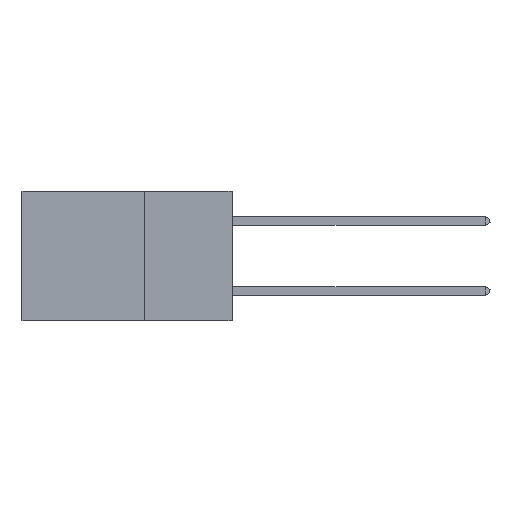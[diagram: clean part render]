
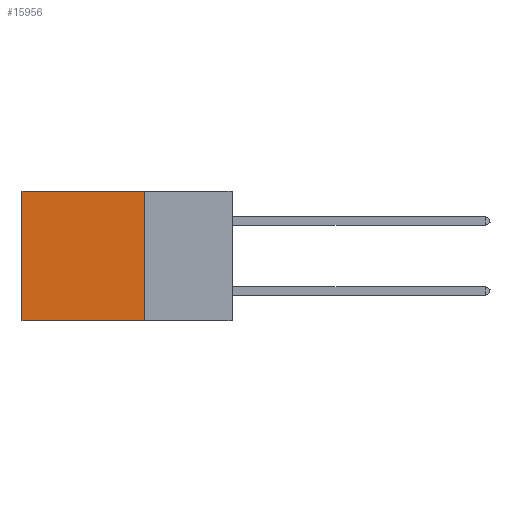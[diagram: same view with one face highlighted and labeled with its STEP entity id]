
A CAD part, left-side view. The second image highlights one B-rep face of the part: STEP entity #15956.
In plain terms, the highlighted planar face has unit normal (-1, 0, 0).
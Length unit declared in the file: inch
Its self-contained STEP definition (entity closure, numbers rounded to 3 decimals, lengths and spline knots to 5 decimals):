
#139 = DIRECTION ( 'NONE',  ( 1., 0., 0. ) ) ;
#235 = CARTESIAN_POINT ( 'NONE',  ( 0.2875, 0.6, -0.37 ) ) ;
#438 = ORIENTED_EDGE ( 'NONE', *, *, #8386, .T. ) ;
#819 = EDGE_CURVE ( 'NONE', #12470, #19053, #14861, .T. ) ;
#3284 = AXIS2_PLACEMENT_3D ( 'NONE', #11725, #139, #13626 ) ;
#4146 = VERTEX_POINT ( 'NONE', #8491 ) ;
#4432 = DIRECTION ( 'NONE',  ( 0., 1., 0. ) ) ;
#5366 = CARTESIAN_POINT ( 'NONE',  ( 0.2875, 0.25, 0. ) ) ;
#5460 = VERTEX_POINT ( 'NONE', #22839 ) ;
#5474 = EDGE_CURVE ( 'NONE', #5460, #4146, #20321, .T. ) ;
#5989 = CARTESIAN_POINT ( 'NONE',  ( 0.2875, 0.25, -0.37 ) ) ;
#6579 = VECTOR ( 'NONE', #16697, 39.37008 ) ;
#8058 = EDGE_CURVE ( 'NONE', #5460, #12470, #16604, .T. ) ;
#8386 = EDGE_CURVE ( 'NONE', #4146, #19053, #14556, .T. ) ;
#8491 = CARTESIAN_POINT ( 'NONE',  ( 0.2875, 0.6, 0. ) ) ;
#9884 = VECTOR ( 'NONE', #20819, 39.37008 ) ;
#10475 = DIRECTION ( 'NONE',  ( 0., 0., -1. ) ) ;
#11123 = FACE_OUTER_BOUND ( 'NONE', #21142, .T. ) ;
#11725 = CARTESIAN_POINT ( 'NONE',  ( 0.2875, 0.25, 0. ) ) ;
#12298 = ORIENTED_EDGE ( 'NONE', *, *, #5474, .T. ) ;
#12470 = VERTEX_POINT ( 'NONE', #18714 ) ;
#13626 = DIRECTION ( 'NONE',  ( 0., 0., -1. ) ) ;
#13695 = ORIENTED_EDGE ( 'NONE', *, *, #819, .F. ) ;
#14556 = LINE ( 'NONE', #17536, #22975 ) ;
#14861 = LINE ( 'NONE', #5989, #9884 ) ;
#15545 = ORIENTED_EDGE ( 'NONE', *, *, #8058, .F. ) ;
#15956 = ADVANCED_FACE ( 'NONE', ( #11123 ), #22588, .F. ) ;
#16145 = VECTOR ( 'NONE', #4432, 39.37008 ) ;
#16604 = LINE ( 'NONE', #5366, #6579 ) ;
#16697 = DIRECTION ( 'NONE',  ( 0., 0., -1. ) ) ;
#17536 = CARTESIAN_POINT ( 'NONE',  ( 0.2875, 0.6, 0. ) ) ;
#17645 = CARTESIAN_POINT ( 'NONE',  ( 0.2875, 0.25, 0. ) ) ;
#18714 = CARTESIAN_POINT ( 'NONE',  ( 0.2875, 0.25, -0.37 ) ) ;
#19053 = VERTEX_POINT ( 'NONE', #235 ) ;
#20321 = LINE ( 'NONE', #17645, #16145 ) ;
#20819 = DIRECTION ( 'NONE',  ( 0., 1., 0. ) ) ;
#21142 = EDGE_LOOP ( 'NONE', ( #438, #13695, #15545, #12298 ) ) ;
#22588 = PLANE ( 'NONE',  #3284 ) ;
#22839 = CARTESIAN_POINT ( 'NONE',  ( 0.2875, 0.25, 0. ) ) ;
#22975 = VECTOR ( 'NONE', #10475, 39.37008 ) ;
